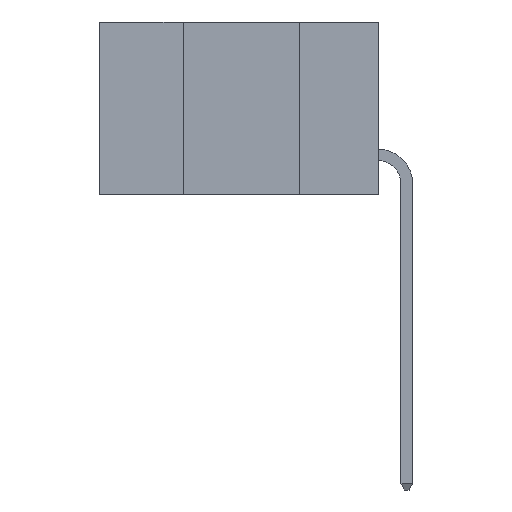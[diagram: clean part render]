
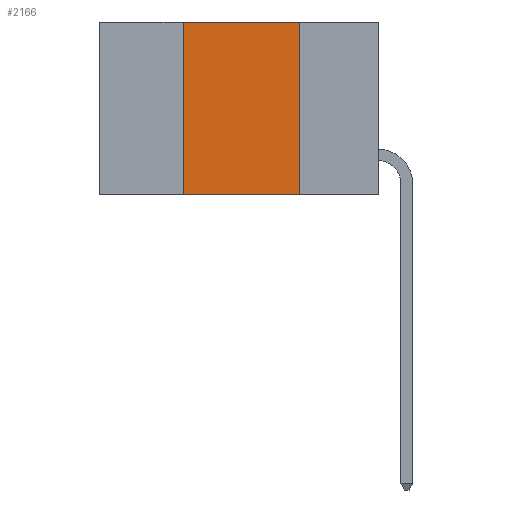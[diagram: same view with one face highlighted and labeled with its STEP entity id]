
A CAD part, left-side view. The second image highlights one B-rep face of the part: STEP entity #2166.
In plain terms, the highlighted planar face has unit normal (-1, 0, 0).
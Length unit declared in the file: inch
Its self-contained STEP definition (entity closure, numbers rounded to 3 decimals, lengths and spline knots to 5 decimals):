
#1569 = VECTOR ( 'NONE', #26246, 39.37008 ) ;
#1771 = EDGE_CURVE ( 'NONE', #18925, #2987, #7942, .T. ) ;
#2166 = ADVANCED_FACE ( 'NONE', ( #14666 ), #4789, .F. ) ;
#2425 = VECTOR ( 'NONE', #18692, 39.37008 ) ;
#2798 = DIRECTION ( 'NONE',  ( 0., 0., 1. ) ) ;
#2971 = CARTESIAN_POINT ( 'NONE',  ( 0., 0.17, 0. ) ) ;
#2987 = VERTEX_POINT ( 'NONE', #2971 ) ;
#3006 = LINE ( 'NONE', #18854, #14007 ) ;
#4193 = DIRECTION ( 'NONE',  ( 0., 0., -1. ) ) ;
#4279 = DIRECTION ( 'NONE',  ( 1., 0., 0. ) ) ;
#4392 = CARTESIAN_POINT ( 'NONE',  ( 0., 0.42, 0. ) ) ;
#4761 = CARTESIAN_POINT ( 'NONE',  ( 0., 0.6, 0. ) ) ;
#4789 = PLANE ( 'NONE',  #10776 ) ;
#5915 = EDGE_CURVE ( 'NONE', #10846, #18925, #22577, .T. ) ;
#5986 = ORIENTED_EDGE ( 'NONE', *, *, #1771, .F. ) ;
#6370 = VECTOR ( 'NONE', #2798, 39.37008 ) ;
#7942 = LINE ( 'NONE', #15004, #2425 ) ;
#8763 = DIRECTION ( 'NONE',  ( 0., 0., -1. ) ) ;
#10167 = CARTESIAN_POINT ( 'NONE',  ( 0., 0.6, -0.37 ) ) ;
#10776 = AXIS2_PLACEMENT_3D ( 'NONE', #4761, #4279, #4193 ) ;
#10846 = VERTEX_POINT ( 'NONE', #20380 ) ;
#12140 = ORIENTED_EDGE ( 'NONE', *, *, #24942, .F. ) ;
#14007 = VECTOR ( 'NONE', #8763, 39.37008 ) ;
#14666 = FACE_OUTER_BOUND ( 'NONE', #24866, .T. ) ;
#14708 = EDGE_CURVE ( 'NONE', #10846, #14939, #22615, .T. ) ;
#14939 = VERTEX_POINT ( 'NONE', #18961 ) ;
#15004 = CARTESIAN_POINT ( 'NONE',  ( 0., 0.6, 0. ) ) ;
#15046 = CARTESIAN_POINT ( 'NONE',  ( 0., 0.42, -0.37 ) ) ;
#18692 = DIRECTION ( 'NONE',  ( 0., -1., 0. ) ) ;
#18854 = CARTESIAN_POINT ( 'NONE',  ( 0., 0.17, -0.37 ) ) ;
#18925 = VERTEX_POINT ( 'NONE', #4392 ) ;
#18961 = CARTESIAN_POINT ( 'NONE',  ( 0., 0.17, -0.37 ) ) ;
#20380 = CARTESIAN_POINT ( 'NONE',  ( 0., 0.42, -0.37 ) ) ;
#20945 = ORIENTED_EDGE ( 'NONE', *, *, #14708, .T. ) ;
#21579 = ORIENTED_EDGE ( 'NONE', *, *, #5915, .F. ) ;
#22577 = LINE ( 'NONE', #15046, #6370 ) ;
#22615 = LINE ( 'NONE', #10167, #1569 ) ;
#24866 = EDGE_LOOP ( 'NONE', ( #12140, #5986, #21579, #20945 ) ) ;
#24942 = EDGE_CURVE ( 'NONE', #2987, #14939, #3006, .T. ) ;
#26246 = DIRECTION ( 'NONE',  ( 0., -1., 0. ) ) ;
